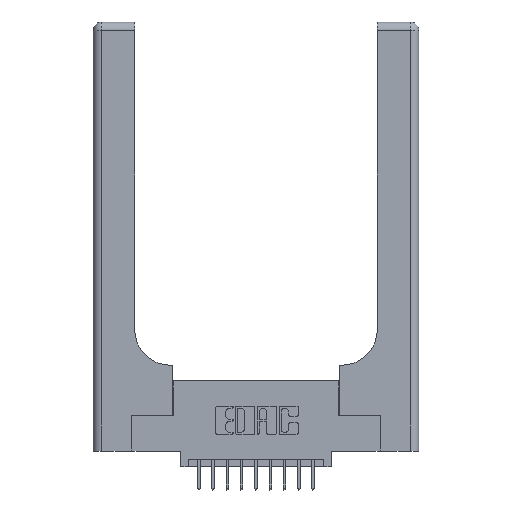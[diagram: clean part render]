
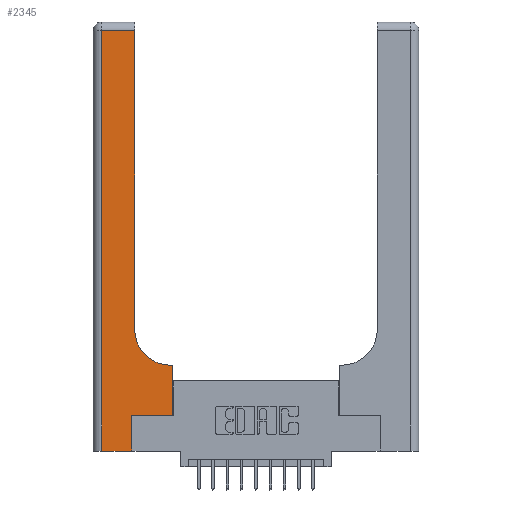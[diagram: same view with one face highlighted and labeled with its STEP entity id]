
A CAD part, top view. The second image highlights one B-rep face of the part: STEP entity #2345.
In plain terms, the highlighted planar face has unit normal (0, 0, 1).
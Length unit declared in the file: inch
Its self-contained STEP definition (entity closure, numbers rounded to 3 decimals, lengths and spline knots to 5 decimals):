
#412 = EDGE_CURVE ( 'NONE', #3943, #4283, #1943, .T. ) ;
#1030 = EDGE_CURVE ( 'NONE', #14042, #15633, #10155, .T. ) ;
#1107 = CARTESIAN_POINT ( 'NONE',  ( 0.269, 0., 0.37 ) ) ;
#1292 = DIRECTION ( 'NONE',  ( 0., 0., -1. ) ) ;
#1387 = LINE ( 'NONE', #9739, #15895 ) ;
#1393 = EDGE_LOOP ( 'NONE', ( #3283, #2754, #2163, #8482, #10256, #15432, #10622, #2790, #10453 ) ) ;
#1719 = DIRECTION ( 'NONE',  ( 0., 0., -1. ) ) ;
#1934 = VERTEX_POINT ( 'NONE', #8372 ) ;
#1943 = LINE ( 'NONE', #12027, #8891 ) ;
#2007 = VECTOR ( 'NONE', #7799, 39.37008 ) ;
#2113 = LINE ( 'NONE', #4855, #11907 ) ;
#2163 = ORIENTED_EDGE ( 'NONE', *, *, #9998, .T. ) ;
#2345 = ADVANCED_FACE ( 'NONE', ( #16187 ), #6481, .F. ) ;
#2361 = CARTESIAN_POINT ( 'NONE',  ( 0.06, 3., 0.37 ) ) ;
#2523 = LINE ( 'NONE', #16852, #11102 ) ;
#2754 = ORIENTED_EDGE ( 'NONE', *, *, #8437, .T. ) ;
#2790 = ORIENTED_EDGE ( 'NONE', *, *, #4491, .T. ) ;
#2921 = EDGE_CURVE ( 'NONE', #1934, #3943, #2523, .T. ) ;
#3283 = ORIENTED_EDGE ( 'NONE', *, *, #4519, .T. ) ;
#3838 = CARTESIAN_POINT ( 'NONE',  ( 0., 2.94, 0.37 ) ) ;
#3943 = VERTEX_POINT ( 'NONE', #1107 ) ;
#4283 = VERTEX_POINT ( 'NONE', #15828 ) ;
#4302 = LINE ( 'NONE', #8270, #5513 ) ;
#4395 = DIRECTION ( 'NONE',  ( 0., 1., 0. ) ) ;
#4491 = EDGE_CURVE ( 'NONE', #5875, #14042, #4302, .T. ) ;
#4519 = EDGE_CURVE ( 'NONE', #15633, #16044, #11043, .T. ) ;
#4855 = CARTESIAN_POINT ( 'NONE',  ( 0.269, 0.25, 0.37 ) ) ;
#5513 = VECTOR ( 'NONE', #16018, 39.37008 ) ;
#5662 = CARTESIAN_POINT ( 'NONE',  ( 0.2915, 2.94, 0.37 ) ) ;
#5875 = VERTEX_POINT ( 'NONE', #16586 ) ;
#6481 = PLANE ( 'NONE',  #10379 ) ;
#7289 = DIRECTION ( 'NONE',  ( 1., 0., 0. ) ) ;
#7429 = CARTESIAN_POINT ( 'NONE',  ( 0.2915, 0.85, 0.37 ) ) ;
#7551 = VERTEX_POINT ( 'NONE', #12800 ) ;
#7799 = DIRECTION ( 'NONE',  ( -1., 0., 0. ) ) ;
#7803 = CARTESIAN_POINT ( 'NONE',  ( 0., 3., 0.37 ) ) ;
#7876 = VERTEX_POINT ( 'NONE', #12961 ) ;
#8205 = EDGE_CURVE ( 'NONE', #7876, #5875, #1387, .T. ) ;
#8270 = CARTESIAN_POINT ( 'NONE',  ( 0.2915, 0.6, 0.37 ) ) ;
#8288 = CARTESIAN_POINT ( 'NONE',  ( 0.5415, 0.85, 0.37 ) ) ;
#8372 = CARTESIAN_POINT ( 'NONE',  ( 0.06, 0., 0.37 ) ) ;
#8437 = EDGE_CURVE ( 'NONE', #16044, #7551, #9574, .T. ) ;
#8482 = ORIENTED_EDGE ( 'NONE', *, *, #2921, .T. ) ;
#8583 = VECTOR ( 'NONE', #4395, 39.37008 ) ;
#8729 = VECTOR ( 'NONE', #15335, 39.37008 ) ;
#8891 = VECTOR ( 'NONE', #15676, 39.37008 ) ;
#9048 = DIRECTION ( 'NONE',  ( 1., 0., 0. ) ) ;
#9574 = LINE ( 'NONE', #3838, #2007 ) ;
#9739 = CARTESIAN_POINT ( 'NONE',  ( 0.5585, 0.25, 0.37 ) ) ;
#9998 = EDGE_CURVE ( 'NONE', #7551, #1934, #12180, .T. ) ;
#10155 = CIRCLE ( 'NONE', #12035, 0.25 ) ;
#10256 = ORIENTED_EDGE ( 'NONE', *, *, #412, .T. ) ;
#10379 = AXIS2_PLACEMENT_3D ( 'NONE', #7803, #1292, #11730 ) ;
#10453 = ORIENTED_EDGE ( 'NONE', *, *, #1030, .T. ) ;
#10622 = ORIENTED_EDGE ( 'NONE', *, *, #8205, .T. ) ;
#11043 = LINE ( 'NONE', #12296, #8583 ) ;
#11102 = VECTOR ( 'NONE', #9048, 39.37008 ) ;
#11730 = DIRECTION ( 'NONE',  ( -1., 0., 0. ) ) ;
#11907 = VECTOR ( 'NONE', #7289, 39.37008 ) ;
#12027 = CARTESIAN_POINT ( 'NONE',  ( 0.269, 0., 0.37 ) ) ;
#12035 = AXIS2_PLACEMENT_3D ( 'NONE', #8288, #1719, #14757 ) ;
#12180 = LINE ( 'NONE', #2361, #8729 ) ;
#12296 = CARTESIAN_POINT ( 'NONE',  ( 0.2915, 3., 0.37 ) ) ;
#12344 = DIRECTION ( 'NONE',  ( 0., 1., 0. ) ) ;
#12800 = CARTESIAN_POINT ( 'NONE',  ( 0.06, 2.94, 0.37 ) ) ;
#12961 = CARTESIAN_POINT ( 'NONE',  ( 0.5585, 0.25, 0.37 ) ) ;
#13197 = CARTESIAN_POINT ( 'NONE',  ( 0.5415, 0.6, 0.37 ) ) ;
#13887 = EDGE_CURVE ( 'NONE', #4283, #7876, #2113, .T. ) ;
#14042 = VERTEX_POINT ( 'NONE', #13197 ) ;
#14757 = DIRECTION ( 'NONE',  ( 1., 0., 0. ) ) ;
#15335 = DIRECTION ( 'NONE',  ( 0., -1., 0. ) ) ;
#15432 = ORIENTED_EDGE ( 'NONE', *, *, #13887, .T. ) ;
#15633 = VERTEX_POINT ( 'NONE', #7429 ) ;
#15676 = DIRECTION ( 'NONE',  ( 0., 1., 0. ) ) ;
#15828 = CARTESIAN_POINT ( 'NONE',  ( 0.269, 0.25, 0.37 ) ) ;
#15895 = VECTOR ( 'NONE', #12344, 39.37008 ) ;
#16018 = DIRECTION ( 'NONE',  ( -1., 0., 0. ) ) ;
#16044 = VERTEX_POINT ( 'NONE', #5662 ) ;
#16187 = FACE_OUTER_BOUND ( 'NONE', #1393, .T. ) ;
#16586 = CARTESIAN_POINT ( 'NONE',  ( 0.5585, 0.6, 0.37 ) ) ;
#16852 = CARTESIAN_POINT ( 'NONE',  ( 0., 0., 0.37 ) ) ;
